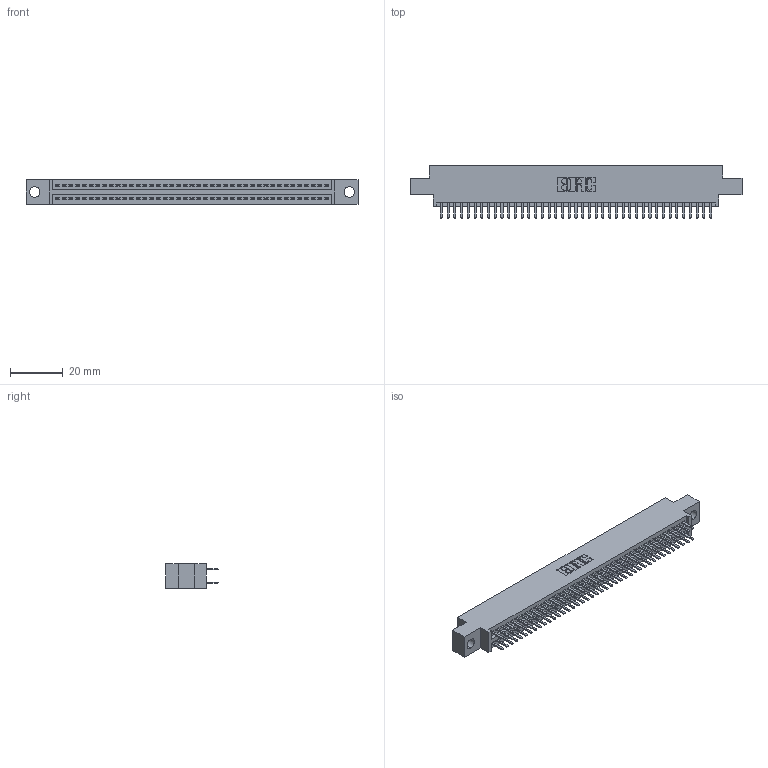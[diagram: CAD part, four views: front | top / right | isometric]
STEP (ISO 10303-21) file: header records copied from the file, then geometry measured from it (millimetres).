
FILE_DESCRIPTION (( 'STEP AP203' ), '1' );
FILE_NAME ('395-082-520-804.STEP', '2018-11-28T06:40:49', ( '' ), ( '' ), 'SwSTEP 2.0', 'SolidWorks 2016', '' );
FILE_SCHEMA (( 'CONFIG_CONTROL_DESIGN' ));
Length unit declared in the file: inch
Products named in the file (3): 345 Part_0.170 Offset - 0.156 Dia-TH; 395-082-520-804; 345-292-001_345-293-120
Assembly tree (83 placements, depth 2):
  395-082-520-804
    345 Part_0.170 Offset - 0.156 Dia-TH
    345-292-001_345-293-120  x82
Bounding box: 125.35 x 19.68 x 9.4 mm (x, y, z)
Volume: 11930 mm3; surface area: 17497.1 mm2
Topology: 83 solids, 83 shells, 4558 faces, 13227 edges, 8598 vertices
Faces by surface type: plane 2954, cylinder 1604
Entity records: 32553 total; most frequent: CARTESIAN_POINT 5472, ORIENTED_EDGE 5394, DIRECTION 4813, EDGE_CURVE 2697, LINE 2397, VECTOR 2397, VERTEX_POINT 1794, AXIS2_PLACEMENT_3D 1208
